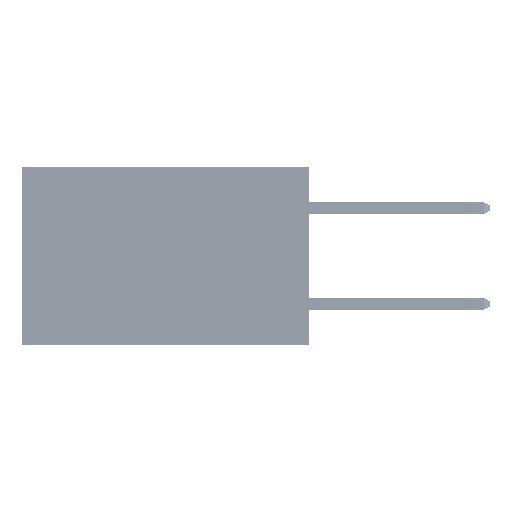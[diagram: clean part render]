
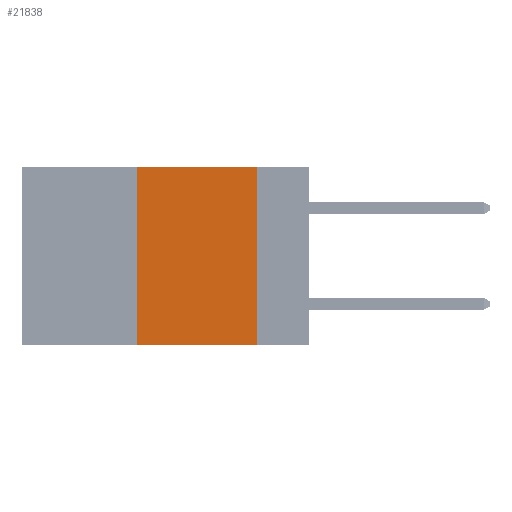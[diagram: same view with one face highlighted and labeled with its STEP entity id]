
A CAD part, left-side view. The second image highlights one B-rep face of the part: STEP entity #21838.
In plain terms, the highlighted planar face has unit normal (-1, 0, 0).
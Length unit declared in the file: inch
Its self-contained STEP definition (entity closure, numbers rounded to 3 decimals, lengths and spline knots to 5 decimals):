
#349 = EDGE_LOOP ( 'NONE', ( #42252, #25853, #30669, #23736 ) ) ;
#1166 = DIRECTION ( 'NONE',  ( 0., 0., 1. ) ) ;
#1748 = DIRECTION ( 'NONE',  ( 0., -1., 0. ) ) ;
#2195 = EDGE_CURVE ( 'NONE', #31581, #45821, #43328, .T. ) ;
#3032 = DIRECTION ( 'NONE',  ( 0., 0., -1. ) ) ;
#3631 = LINE ( 'NONE', #16666, #13904 ) ;
#5669 = CARTESIAN_POINT ( 'NONE',  ( 0., 0.36, -0.37 ) ) ;
#10663 = AXIS2_PLACEMENT_3D ( 'NONE', #49227, #40974, #3032 ) ;
#12966 = VECTOR ( 'NONE', #1748, 39.37008 ) ;
#13904 = VECTOR ( 'NONE', #1166, 39.37008 ) ;
#13936 = VERTEX_POINT ( 'NONE', #5669 ) ;
#15476 = FACE_OUTER_BOUND ( 'NONE', #349, .T. ) ;
#16666 = CARTESIAN_POINT ( 'NONE',  ( 0., 0.36, 0. ) ) ;
#16697 = DIRECTION ( 'NONE',  ( 0., -1., 0. ) ) ;
#20587 = CARTESIAN_POINT ( 'NONE',  ( 0., 0.6, 0. ) ) ;
#21838 = ADVANCED_FACE ( 'NONE', ( #15476 ), #22260, .F. ) ;
#21893 = CARTESIAN_POINT ( 'NONE',  ( 0., 0.36, 0. ) ) ;
#22260 = PLANE ( 'NONE',  #10663 ) ;
#23736 = ORIENTED_EDGE ( 'NONE', *, *, #27226, .T. ) ;
#24585 = DIRECTION ( 'NONE',  ( 0., 0., -1. ) ) ;
#25853 = ORIENTED_EDGE ( 'NONE', *, *, #27749, .F. ) ;
#26497 = VECTOR ( 'NONE', #24585, 39.37008 ) ;
#27226 = EDGE_CURVE ( 'NONE', #13936, #45821, #41298, .T. ) ;
#27749 = EDGE_CURVE ( 'NONE', #44661, #31581, #32333, .T. ) ;
#28486 = CARTESIAN_POINT ( 'NONE',  ( 0., 0.11, 0. ) ) ;
#29860 = CARTESIAN_POINT ( 'NONE',  ( 0., 0.11, -0.37 ) ) ;
#30669 = ORIENTED_EDGE ( 'NONE', *, *, #30722, .F. ) ;
#30722 = EDGE_CURVE ( 'NONE', #13936, #44661, #3631, .T. ) ;
#31581 = VERTEX_POINT ( 'NONE', #40870 ) ;
#32333 = LINE ( 'NONE', #20587, #49760 ) ;
#40870 = CARTESIAN_POINT ( 'NONE',  ( 0., 0.11, 0. ) ) ;
#40974 = DIRECTION ( 'NONE',  ( 1., 0., 0. ) ) ;
#41298 = LINE ( 'NONE', #44242, #12966 ) ;
#42252 = ORIENTED_EDGE ( 'NONE', *, *, #2195, .F. ) ;
#43328 = LINE ( 'NONE', #28486, #26497 ) ;
#44242 = CARTESIAN_POINT ( 'NONE',  ( 0., 0.6, -0.37 ) ) ;
#44661 = VERTEX_POINT ( 'NONE', #21893 ) ;
#45821 = VERTEX_POINT ( 'NONE', #29860 ) ;
#49227 = CARTESIAN_POINT ( 'NONE',  ( 0., 0.6, 0. ) ) ;
#49760 = VECTOR ( 'NONE', #16697, 39.37008 ) ;
